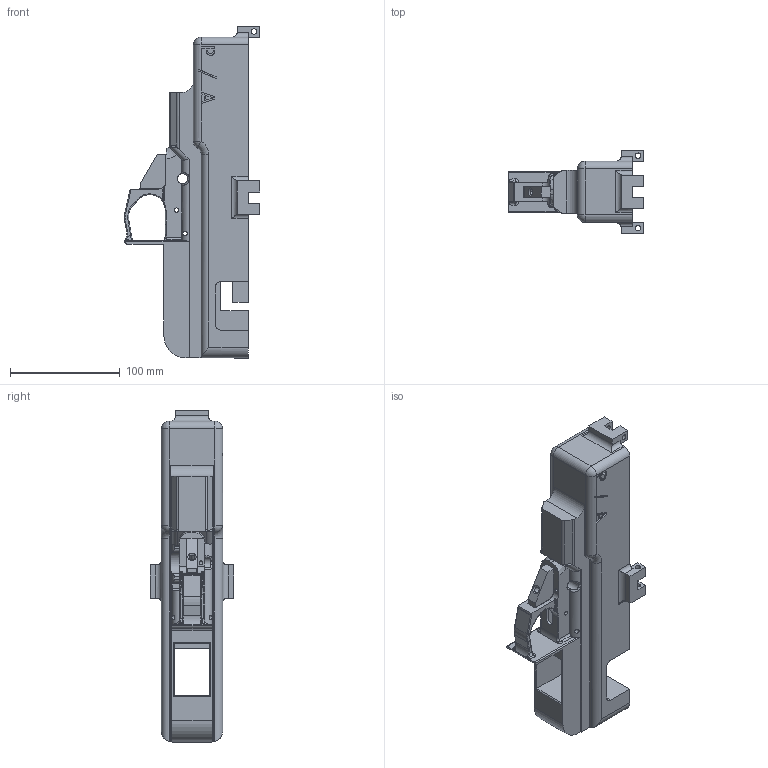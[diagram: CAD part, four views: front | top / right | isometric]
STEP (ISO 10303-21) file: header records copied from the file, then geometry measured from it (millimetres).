
FILE_DESCRIPTION (( 'STEP AP214' ), '1' );
FILE_NAME ('Frame_complete.STEP', '2013-09-23T23:59:50', ( '' ), ( '' ), 'SwSTEP 2.0', 'SolidWorks 2013', '' );
FILE_SCHEMA (( 'AUTOMOTIVE_DESIGN' ));
Length unit declared in the file: millimetre
Products named in the file (1): Frame_complete
Bounding box: 123.33 x 76.25 x 303 mm (x, y, z)
Volume: 508932.3 mm3; surface area: 121767 mm2
Topology: 1 solids, 1 shells, 399 faces, 1092 edges, 689 vertices
Faces by surface type: plane 169, cylinder 153, bspline 58, torus 11, cone 4, sphere 4
Entity records: 15831 total; most frequent: CARTESIAN_POINT 6110, ORIENTED_EDGE 2176, DIRECTION 1846, EDGE_CURVE 1088, VERTEX_POINT 689, AXIS2_PLACEMENT_3D 618, VECTOR 610, LINE 610
